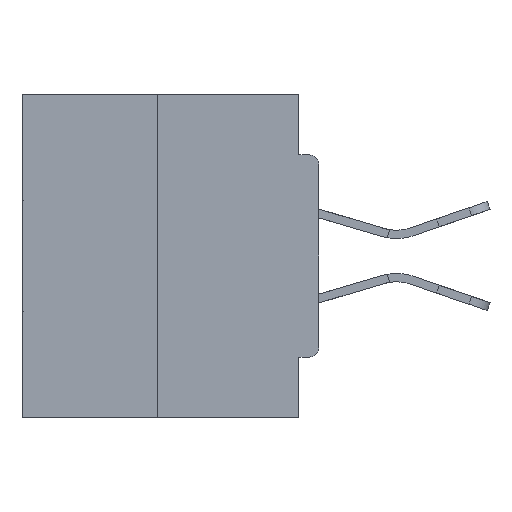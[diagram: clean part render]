
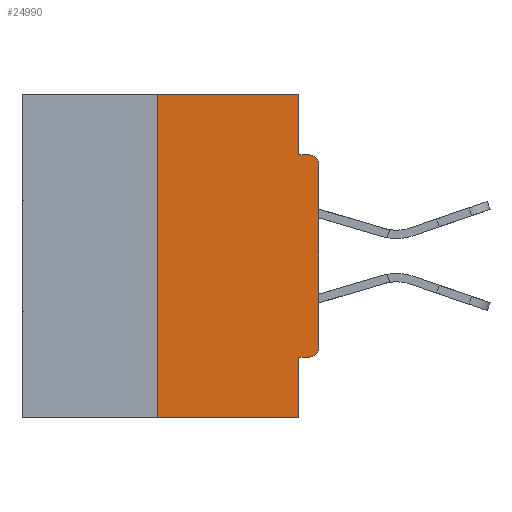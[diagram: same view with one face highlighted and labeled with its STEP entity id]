
A CAD part, left-side view. The second image highlights one B-rep face of the part: STEP entity #24990.
In plain terms, the highlighted planar face has unit normal (-1, 0, 0).
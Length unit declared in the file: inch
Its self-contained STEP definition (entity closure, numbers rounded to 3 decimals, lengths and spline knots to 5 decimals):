
#120 = CARTESIAN_POINT ( 'NONE',  ( 0., 0., -0.1085 ) ) ;
#1050 = CARTESIAN_POINT ( 'NONE',  ( 0., 0.031, 0. ) ) ;
#2099 = AXIS2_PLACEMENT_3D ( 'NONE', #34171, #28569, #12338 ) ;
#2847 = PLANE ( 'NONE',  #8871 ) ;
#3117 = CARTESIAN_POINT ( 'NONE',  ( 0., 0.015, -0.1085 ) ) ;
#3141 = VERTEX_POINT ( 'NONE', #16192 ) ;
#3817 = VECTOR ( 'NONE', #11382, 39.37008 ) ;
#4675 = VERTEX_POINT ( 'NONE', #38476 ) ;
#4814 = CARTESIAN_POINT ( 'NONE',  ( 0., 0.031, 0. ) ) ;
#5215 = VERTEX_POINT ( 'NONE', #1050 ) ;
#5396 = CARTESIAN_POINT ( 'NONE',  ( 0., 0., 0. ) ) ;
#5543 = VECTOR ( 'NONE', #30195, 39.37008 ) ;
#5629 = VECTOR ( 'NONE', #23863, 39.37008 ) ;
#5645 = DIRECTION ( 'NONE',  ( 0., 0., -1. ) ) ;
#5905 = VERTEX_POINT ( 'NONE', #120 ) ;
#6445 = DIRECTION ( 'NONE',  ( 0., 0., -1. ) ) ;
#6508 = EDGE_CURVE ( 'NONE', #33179, #4675, #31777, .T. ) ;
#7277 = VECTOR ( 'NONE', #21412, 39.37008 ) ;
#7575 = EDGE_CURVE ( 'NONE', #31578, #4675, #27287, .T. ) ;
#7616 = ORIENTED_EDGE ( 'NONE', *, *, #33967, .T. ) ;
#8871 = AXIS2_PLACEMENT_3D ( 'NONE', #15427, #29615, #10669 ) ;
#9092 = ORIENTED_EDGE ( 'NONE', *, *, #21628, .T. ) ;
#9117 = DIRECTION ( 'NONE',  ( -1., 0., 0. ) ) ;
#9843 = VERTEX_POINT ( 'NONE', #23855 ) ;
#10565 = VECTOR ( 'NONE', #16683, 39.37008 ) ;
#10587 = CARTESIAN_POINT ( 'NONE',  ( 0., 0.25, -0.5 ) ) ;
#10669 = DIRECTION ( 'NONE',  ( 0., 0., -1. ) ) ;
#11382 = DIRECTION ( 'NONE',  ( 0., 0., 1. ) ) ;
#12152 = CARTESIAN_POINT ( 'NONE',  ( 0., 0., -0.4065 ) ) ;
#12338 = DIRECTION ( 'NONE',  ( 0., 0., -1. ) ) ;
#13397 = EDGE_CURVE ( 'NONE', #9843, #30316, #39389, .T. ) ;
#13828 = ORIENTED_EDGE ( 'NONE', *, *, #7575, .T. ) ;
#14010 = CARTESIAN_POINT ( 'NONE',  ( 0., 0.015, -0.0935 ) ) ;
#14608 = CIRCLE ( 'NONE', #2099, 0.015 ) ;
#15003 = EDGE_CURVE ( 'NONE', #37419, #33179, #36892, .T. ) ;
#15427 = CARTESIAN_POINT ( 'NONE',  ( 0., 0.46, 0. ) ) ;
#16192 = CARTESIAN_POINT ( 'NONE',  ( 0., 0.25, 0. ) ) ;
#16334 = DIRECTION ( 'NONE',  ( 0., 0., -1. ) ) ;
#16683 = DIRECTION ( 'NONE',  ( 0., -1., 0. ) ) ;
#16936 = CARTESIAN_POINT ( 'NONE',  ( 0., 0.031, -0.4065 ) ) ;
#17675 = ORIENTED_EDGE ( 'NONE', *, *, #24060, .F. ) ;
#18873 = CIRCLE ( 'NONE', #35355, 0.015 ) ;
#19192 = CARTESIAN_POINT ( 'NONE',  ( 0., 0.031, -0.5 ) ) ;
#20561 = ORIENTED_EDGE ( 'NONE', *, *, #13397, .F. ) ;
#20569 = LINE ( 'NONE', #32341, #5629 ) ;
#21412 = DIRECTION ( 'NONE',  ( 0., 1., 0. ) ) ;
#21424 = EDGE_CURVE ( 'NONE', #24105, #5905, #30524, .T. ) ;
#21628 = EDGE_CURVE ( 'NONE', #5905, #30316, #18873, .T. ) ;
#21908 = DIRECTION ( 'NONE',  ( 0., -1., 0. ) ) ;
#22190 = ORIENTED_EDGE ( 'NONE', *, *, #15003, .F. ) ;
#22522 = CARTESIAN_POINT ( 'NONE',  ( 0., 0.46, 0. ) ) ;
#23358 = VECTOR ( 'NONE', #21908, 39.37008 ) ;
#23855 = CARTESIAN_POINT ( 'NONE',  ( 0., 0.031, -0.0935 ) ) ;
#23863 = DIRECTION ( 'NONE',  ( 0., 0., 1. ) ) ;
#23901 = VECTOR ( 'NONE', #16334, 39.37008 ) ;
#24060 = EDGE_CURVE ( 'NONE', #3141, #5215, #31608, .T. ) ;
#24105 = VERTEX_POINT ( 'NONE', #37807 ) ;
#24363 = EDGE_LOOP ( 'NONE', ( #17675, #32537, #13828, #29102, #22190, #7616, #27430, #9092, #20561, #40582 ) ) ;
#24990 = ADVANCED_FACE ( 'NONE', ( #31294 ), #2847, .F. ) ;
#27287 = LINE ( 'NONE', #39919, #5543 ) ;
#27430 = ORIENTED_EDGE ( 'NONE', *, *, #21424, .T. ) ;
#28569 = DIRECTION ( 'NONE',  ( -1., 0., 0. ) ) ;
#29102 = ORIENTED_EDGE ( 'NONE', *, *, #6508, .F. ) ;
#29615 = DIRECTION ( 'NONE',  ( 1., 0., 0. ) ) ;
#30195 = DIRECTION ( 'NONE',  ( 0., -1., 0. ) ) ;
#30316 = VERTEX_POINT ( 'NONE', #14010 ) ;
#30524 = LINE ( 'NONE', #5396, #3817 ) ;
#31294 = FACE_OUTER_BOUND ( 'NONE', #24363, .T. ) ;
#31578 = VERTEX_POINT ( 'NONE', #10587 ) ;
#31608 = LINE ( 'NONE', #22522, #23358 ) ;
#31777 = LINE ( 'NONE', #19192, #23901 ) ;
#32341 = CARTESIAN_POINT ( 'NONE',  ( 0., 0.25, 0. ) ) ;
#32350 = CARTESIAN_POINT ( 'NONE',  ( 0., 0., -0.0935 ) ) ;
#32537 = ORIENTED_EDGE ( 'NONE', *, *, #37168, .F. ) ;
#33179 = VERTEX_POINT ( 'NONE', #16936 ) ;
#33462 = LINE ( 'NONE', #4814, #39272 ) ;
#33967 = EDGE_CURVE ( 'NONE', #37419, #24105, #14608, .T. ) ;
#33973 = CARTESIAN_POINT ( 'NONE',  ( 0., 0.015, -0.4065 ) ) ;
#34171 = CARTESIAN_POINT ( 'NONE',  ( 0., 0.015, -0.3915 ) ) ;
#35355 = AXIS2_PLACEMENT_3D ( 'NONE', #3117, #9117, #6445 ) ;
#36892 = LINE ( 'NONE', #12152, #7277 ) ;
#37168 = EDGE_CURVE ( 'NONE', #31578, #3141, #20569, .T. ) ;
#37419 = VERTEX_POINT ( 'NONE', #33973 ) ;
#37807 = CARTESIAN_POINT ( 'NONE',  ( 0., 0., -0.3915 ) ) ;
#38281 = EDGE_CURVE ( 'NONE', #5215, #9843, #33462, .T. ) ;
#38476 = CARTESIAN_POINT ( 'NONE',  ( 0., 0.031, -0.5 ) ) ;
#39272 = VECTOR ( 'NONE', #5645, 39.37008 ) ;
#39389 = LINE ( 'NONE', #32350, #10565 ) ;
#39919 = CARTESIAN_POINT ( 'NONE',  ( 0., 0.46, -0.5 ) ) ;
#40582 = ORIENTED_EDGE ( 'NONE', *, *, #38281, .F. ) ;
